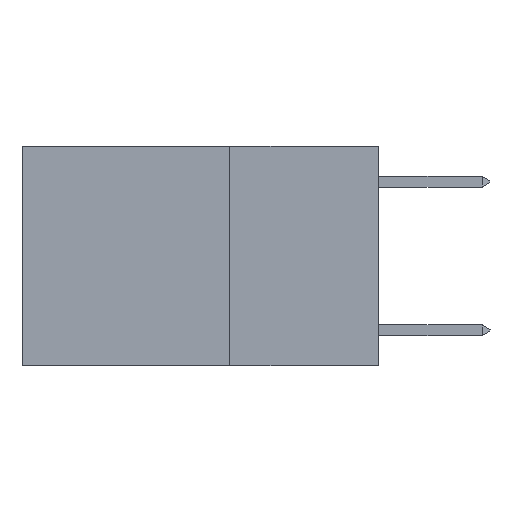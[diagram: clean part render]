
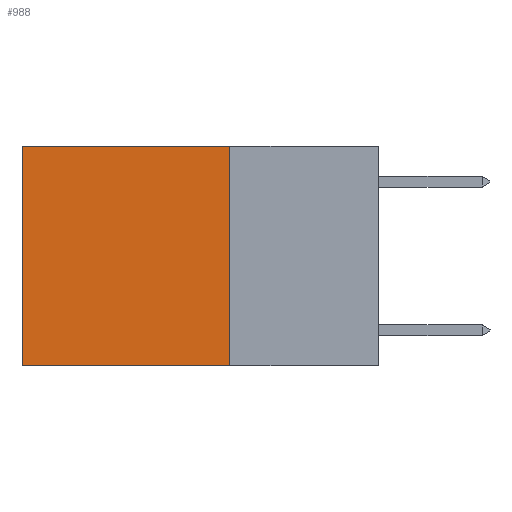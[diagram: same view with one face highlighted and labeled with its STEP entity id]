
A CAD part, left-side view. The second image highlights one B-rep face of the part: STEP entity #988.
In plain terms, the highlighted planar face has unit normal (-1, 0, 0).
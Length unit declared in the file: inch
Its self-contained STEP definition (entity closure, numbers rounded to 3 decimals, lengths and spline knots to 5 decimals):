
#152 = PLANE ( 'NONE',  #10795 ) ;
#492 = ORIENTED_EDGE ( 'NONE', *, *, #14976, .T. ) ;
#988 = ADVANCED_FACE ( 'NONE', ( #3633 ), #152, .F. ) ;
#1248 = VERTEX_POINT ( 'NONE', #10700 ) ;
#1284 = CARTESIAN_POINT ( 'NONE',  ( 0.2625, 0.25, -0.37 ) ) ;
#1972 = CARTESIAN_POINT ( 'NONE',  ( 0.2625, 0.25, -0.37 ) ) ;
#2027 = CARTESIAN_POINT ( 'NONE',  ( 0.2625, 0.25, 0. ) ) ;
#2519 = VECTOR ( 'NONE', #10993, 39.37008 ) ;
#2547 = VECTOR ( 'NONE', #8706, 39.37008 ) ;
#2684 = DIRECTION ( 'NONE',  ( 1., 0., 0. ) ) ;
#2892 = LINE ( 'NONE', #1284, #2519 ) ;
#3383 = ORIENTED_EDGE ( 'NONE', *, *, #10450, .F. ) ;
#3544 = CARTESIAN_POINT ( 'NONE',  ( 0.2625, 0.6, 0. ) ) ;
#3633 = FACE_OUTER_BOUND ( 'NONE', #3797, .T. ) ;
#3797 = EDGE_LOOP ( 'NONE', ( #9196, #3383, #9552, #492 ) ) ;
#3798 = CARTESIAN_POINT ( 'NONE',  ( 0.2625, 0.25, 0. ) ) ;
#4296 = LINE ( 'NONE', #3544, #7342 ) ;
#4624 = EDGE_CURVE ( 'NONE', #12823, #10757, #14596, .T. ) ;
#5113 = LINE ( 'NONE', #6047, #10956 ) ;
#6047 = CARTESIAN_POINT ( 'NONE',  ( 0.2625, 0.25, 0. ) ) ;
#7342 = VECTOR ( 'NONE', #10509, 39.37008 ) ;
#7497 = EDGE_CURVE ( 'NONE', #8837, #1248, #4296, .T. ) ;
#8391 = DIRECTION ( 'NONE',  ( 0., 1., 0. ) ) ;
#8706 = DIRECTION ( 'NONE',  ( 0., 0., -1. ) ) ;
#8837 = VERTEX_POINT ( 'NONE', #9502 ) ;
#9196 = ORIENTED_EDGE ( 'NONE', *, *, #7497, .T. ) ;
#9502 = CARTESIAN_POINT ( 'NONE',  ( 0.2625, 0.6, 0. ) ) ;
#9552 = ORIENTED_EDGE ( 'NONE', *, *, #4624, .F. ) ;
#10450 = EDGE_CURVE ( 'NONE', #10757, #1248, #2892, .T. ) ;
#10509 = DIRECTION ( 'NONE',  ( 0., 0., -1. ) ) ;
#10700 = CARTESIAN_POINT ( 'NONE',  ( 0.2625, 0.6, -0.37 ) ) ;
#10757 = VERTEX_POINT ( 'NONE', #1972 ) ;
#10795 = AXIS2_PLACEMENT_3D ( 'NONE', #3798, #2684, #10826 ) ;
#10826 = DIRECTION ( 'NONE',  ( 0., 0., -1. ) ) ;
#10956 = VECTOR ( 'NONE', #8391, 39.37008 ) ;
#10993 = DIRECTION ( 'NONE',  ( 0., 1., 0. ) ) ;
#12228 = CARTESIAN_POINT ( 'NONE',  ( 0.2625, 0.25, 0. ) ) ;
#12823 = VERTEX_POINT ( 'NONE', #2027 ) ;
#14596 = LINE ( 'NONE', #12228, #2547 ) ;
#14976 = EDGE_CURVE ( 'NONE', #12823, #8837, #5113, .T. ) ;
